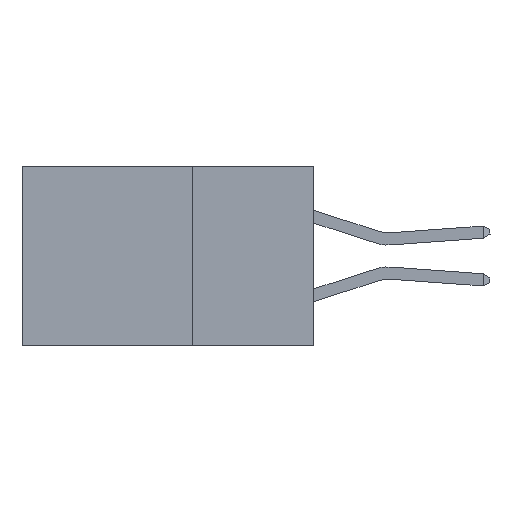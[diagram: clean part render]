
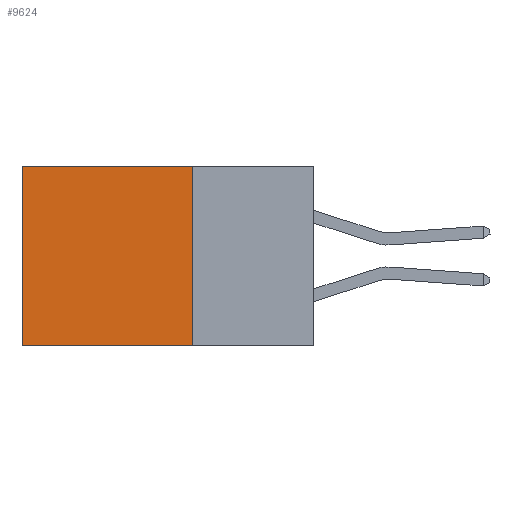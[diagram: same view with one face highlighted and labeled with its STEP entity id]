
A CAD part, left-side view. The second image highlights one B-rep face of the part: STEP entity #9624.
In plain terms, the highlighted planar face has unit normal (-1, 0, 0).
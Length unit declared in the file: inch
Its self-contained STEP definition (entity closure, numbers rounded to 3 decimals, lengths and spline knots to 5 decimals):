
#707 = EDGE_CURVE ( 'NONE', #3349, #11208, #13103, .T. ) ;
#876 = EDGE_LOOP ( 'NONE', ( #9685, #883, #11413, #10110 ) ) ;
#883 = ORIENTED_EDGE ( 'NONE', *, *, #707, .F. ) ;
#1153 = EDGE_CURVE ( 'NONE', #6110, #3349, #2263, .T. ) ;
#1930 = VECTOR ( 'NONE', #5354, 39.37008 ) ;
#2263 = LINE ( 'NONE', #6225, #1930 ) ;
#2530 = CARTESIAN_POINT ( 'NONE',  ( 0.2875, 0.25, 0. ) ) ;
#3107 = LINE ( 'NONE', #7345, #3915 ) ;
#3349 = VERTEX_POINT ( 'NONE', #10847 ) ;
#3666 = FACE_OUTER_BOUND ( 'NONE', #876, .T. ) ;
#3720 = DIRECTION ( 'NONE',  ( 0., 1., 0. ) ) ;
#3915 = VECTOR ( 'NONE', #12370, 39.37008 ) ;
#5178 = EDGE_CURVE ( 'NONE', #6110, #8640, #5313, .T. ) ;
#5313 = LINE ( 'NONE', #8496, #7116 ) ;
#5354 = DIRECTION ( 'NONE',  ( 0., 0., -1. ) ) ;
#5816 = DIRECTION ( 'NONE',  ( 0., 0., -1. ) ) ;
#6110 = VERTEX_POINT ( 'NONE', #7949 ) ;
#6225 = CARTESIAN_POINT ( 'NONE',  ( 0.2875, 0.25, 0. ) ) ;
#6801 = CARTESIAN_POINT ( 'NONE',  ( 0.2875, 0.25, -0.37 ) ) ;
#7116 = VECTOR ( 'NONE', #9441, 39.37008 ) ;
#7345 = CARTESIAN_POINT ( 'NONE',  ( 0.2875, 0.6, 0. ) ) ;
#7510 = EDGE_CURVE ( 'NONE', #8640, #11208, #3107, .T. ) ;
#7949 = CARTESIAN_POINT ( 'NONE',  ( 0.2875, 0.25, 0. ) ) ;
#8496 = CARTESIAN_POINT ( 'NONE',  ( 0.2875, 0.25, 0. ) ) ;
#8640 = VERTEX_POINT ( 'NONE', #12869 ) ;
#9441 = DIRECTION ( 'NONE',  ( 0., 1., 0. ) ) ;
#9624 = ADVANCED_FACE ( 'NONE', ( #3666 ), #10954, .F. ) ;
#9685 = ORIENTED_EDGE ( 'NONE', *, *, #7510, .T. ) ;
#10110 = ORIENTED_EDGE ( 'NONE', *, *, #5178, .T. ) ;
#10319 = VECTOR ( 'NONE', #3720, 39.37008 ) ;
#10847 = CARTESIAN_POINT ( 'NONE',  ( 0.2875, 0.25, -0.37 ) ) ;
#10954 = PLANE ( 'NONE',  #12758 ) ;
#11208 = VERTEX_POINT ( 'NONE', #13207 ) ;
#11413 = ORIENTED_EDGE ( 'NONE', *, *, #1153, .F. ) ;
#11716 = DIRECTION ( 'NONE',  ( 1., 0., 0. ) ) ;
#12370 = DIRECTION ( 'NONE',  ( 0., 0., -1. ) ) ;
#12758 = AXIS2_PLACEMENT_3D ( 'NONE', #2530, #11716, #5816 ) ;
#12869 = CARTESIAN_POINT ( 'NONE',  ( 0.2875, 0.6, 0. ) ) ;
#13103 = LINE ( 'NONE', #6801, #10319 ) ;
#13207 = CARTESIAN_POINT ( 'NONE',  ( 0.2875, 0.6, -0.37 ) ) ;
